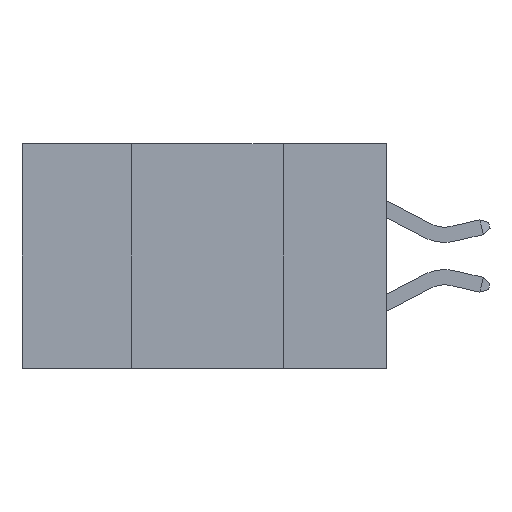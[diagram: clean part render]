
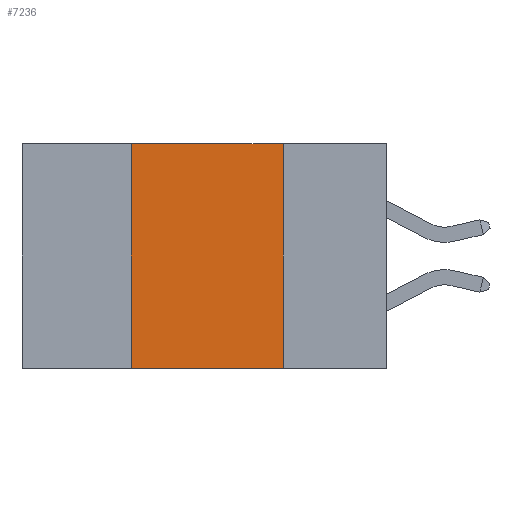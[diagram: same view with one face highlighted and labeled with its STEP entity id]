
A CAD part, left-side view. The second image highlights one B-rep face of the part: STEP entity #7236.
In plain terms, the highlighted planar face has unit normal (-1, 0, 0).
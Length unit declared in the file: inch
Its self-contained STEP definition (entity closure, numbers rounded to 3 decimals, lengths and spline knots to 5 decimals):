
#102 = VECTOR ( 'NONE', #13545, 39.37008 ) ;
#1353 = EDGE_CURVE ( 'NONE', #7088, #8510, #7974, .T. ) ;
#1694 = CARTESIAN_POINT ( 'NONE',  ( 0., 0.42, 0. ) ) ;
#1760 = VECTOR ( 'NONE', #7138, 39.37008 ) ;
#2311 = CARTESIAN_POINT ( 'NONE',  ( 0., 0.17, -0.37 ) ) ;
#2479 = FACE_OUTER_BOUND ( 'NONE', #10573, .T. ) ;
#2770 = CARTESIAN_POINT ( 'NONE',  ( 0., 0.6, 0. ) ) ;
#2953 = DIRECTION ( 'NONE',  ( 0., 0., -1. ) ) ;
#3563 = AXIS2_PLACEMENT_3D ( 'NONE', #2770, #3848, #6421 ) ;
#3848 = DIRECTION ( 'NONE',  ( 1., 0., 0. ) ) ;
#3970 = LINE ( 'NONE', #10649, #10976 ) ;
#4028 = EDGE_CURVE ( 'NONE', #7088, #7670, #10994, .T. ) ;
#4301 = EDGE_CURVE ( 'NONE', #11969, #7670, #3970, .T. ) ;
#4693 = CARTESIAN_POINT ( 'NONE',  ( 0., 0.6, 0. ) ) ;
#4789 = CARTESIAN_POINT ( 'NONE',  ( 0., 0.42, -0.37 ) ) ;
#5800 = EDGE_CURVE ( 'NONE', #8510, #11969, #6952, .T. ) ;
#6421 = DIRECTION ( 'NONE',  ( 0., 0., -1. ) ) ;
#6952 = LINE ( 'NONE', #4693, #102 ) ;
#7088 = VERTEX_POINT ( 'NONE', #4789 ) ;
#7138 = DIRECTION ( 'NONE',  ( 0., -1., 0. ) ) ;
#7236 = ADVANCED_FACE ( 'NONE', ( #2479 ), #14213, .F. ) ;
#7670 = VERTEX_POINT ( 'NONE', #2311 ) ;
#7974 = LINE ( 'NONE', #1694, #8797 ) ;
#8228 = CARTESIAN_POINT ( 'NONE',  ( 0., 0.42, 0. ) ) ;
#8510 = VERTEX_POINT ( 'NONE', #8228 ) ;
#8572 = ORIENTED_EDGE ( 'NONE', *, *, #4301, .F. ) ;
#8797 = VECTOR ( 'NONE', #11911, 39.37008 ) ;
#9742 = CARTESIAN_POINT ( 'NONE',  ( 0., 0.6, -0.37 ) ) ;
#10573 = EDGE_LOOP ( 'NONE', ( #8572, #12320, #15447, #12927 ) ) ;
#10649 = CARTESIAN_POINT ( 'NONE',  ( 0., 0.17, 0. ) ) ;
#10976 = VECTOR ( 'NONE', #2953, 39.37008 ) ;
#10994 = LINE ( 'NONE', #9742, #1760 ) ;
#11911 = DIRECTION ( 'NONE',  ( 0., 0., 1. ) ) ;
#11969 = VERTEX_POINT ( 'NONE', #12586 ) ;
#12320 = ORIENTED_EDGE ( 'NONE', *, *, #5800, .F. ) ;
#12586 = CARTESIAN_POINT ( 'NONE',  ( 0., 0.17, 0. ) ) ;
#12927 = ORIENTED_EDGE ( 'NONE', *, *, #4028, .T. ) ;
#13545 = DIRECTION ( 'NONE',  ( 0., -1., 0. ) ) ;
#14213 = PLANE ( 'NONE',  #3563 ) ;
#15447 = ORIENTED_EDGE ( 'NONE', *, *, #1353, .F. ) ;
